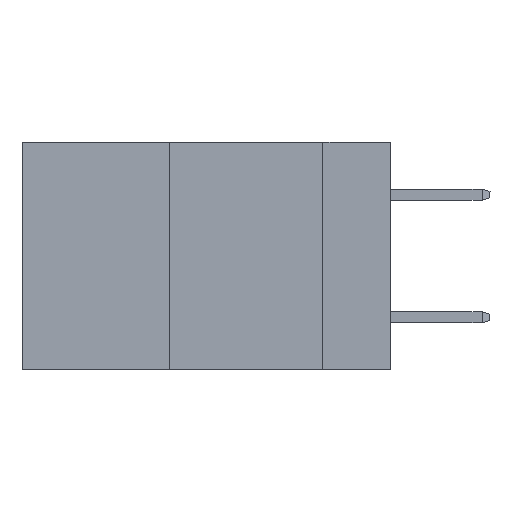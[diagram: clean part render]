
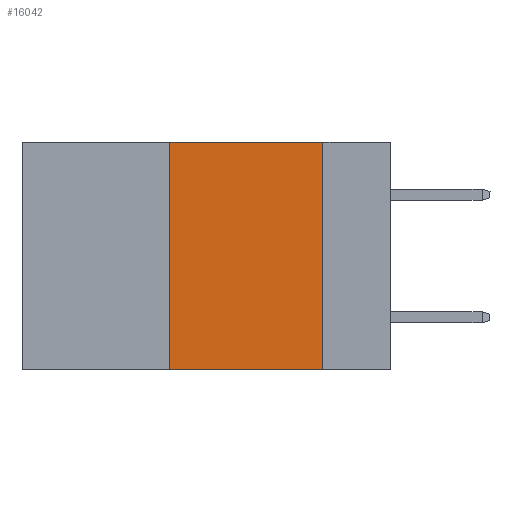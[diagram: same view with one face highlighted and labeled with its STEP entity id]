
A CAD part, left-side view. The second image highlights one B-rep face of the part: STEP entity #16042.
In plain terms, the highlighted planar face has unit normal (-1, 0, 0).
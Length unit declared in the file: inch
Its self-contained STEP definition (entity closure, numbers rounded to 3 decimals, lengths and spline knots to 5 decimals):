
#69 = AXIS2_PLACEMENT_3D ( 'NONE', #8861, #10184, #2370 ) ;
#416 = DIRECTION ( 'NONE',  ( 0., -1., 0. ) ) ;
#794 = CARTESIAN_POINT ( 'NONE',  ( 0., 0.6, -0.37 ) ) ;
#1699 = CARTESIAN_POINT ( 'NONE',  ( 0., 0.36, 0. ) ) ;
#1700 = CARTESIAN_POINT ( 'NONE',  ( 0., 0.36, 0. ) ) ;
#2370 = DIRECTION ( 'NONE',  ( 0., 0., -1. ) ) ;
#2423 = VERTEX_POINT ( 'NONE', #6934 ) ;
#4205 = EDGE_CURVE ( 'NONE', #4821, #9340, #15015, .T. ) ;
#4734 = FACE_OUTER_BOUND ( 'NONE', #6098, .T. ) ;
#4821 = VERTEX_POINT ( 'NONE', #1699 ) ;
#5469 = EDGE_CURVE ( 'NONE', #9340, #2423, #13984, .T. ) ;
#5676 = EDGE_CURVE ( 'NONE', #10452, #2423, #8193, .T. ) ;
#6098 = EDGE_LOOP ( 'NONE', ( #7276, #10750, #9312, #6688 ) ) ;
#6688 = ORIENTED_EDGE ( 'NONE', *, *, #5676, .T. ) ;
#6934 = CARTESIAN_POINT ( 'NONE',  ( 0., 0.11, -0.37 ) ) ;
#7276 = ORIENTED_EDGE ( 'NONE', *, *, #5469, .F. ) ;
#7585 = VECTOR ( 'NONE', #15922, 39.37008 ) ;
#7773 = VECTOR ( 'NONE', #10014, 39.37008 ) ;
#8193 = LINE ( 'NONE', #794, #7773 ) ;
#8861 = CARTESIAN_POINT ( 'NONE',  ( 0., 0.6, 0. ) ) ;
#9312 = ORIENTED_EDGE ( 'NONE', *, *, #10971, .F. ) ;
#9340 = VERTEX_POINT ( 'NONE', #12831 ) ;
#9648 = CARTESIAN_POINT ( 'NONE',  ( 0., 0.6, 0. ) ) ;
#9767 = CARTESIAN_POINT ( 'NONE',  ( 0., 0.36, -0.37 ) ) ;
#9960 = LINE ( 'NONE', #1700, #10378 ) ;
#10014 = DIRECTION ( 'NONE',  ( 0., -1., 0. ) ) ;
#10184 = DIRECTION ( 'NONE',  ( 1., 0., 0. ) ) ;
#10378 = VECTOR ( 'NONE', #15835, 39.37008 ) ;
#10452 = VERTEX_POINT ( 'NONE', #9767 ) ;
#10750 = ORIENTED_EDGE ( 'NONE', *, *, #4205, .F. ) ;
#10971 = EDGE_CURVE ( 'NONE', #10452, #4821, #9960, .T. ) ;
#12091 = VECTOR ( 'NONE', #416, 39.37008 ) ;
#12831 = CARTESIAN_POINT ( 'NONE',  ( 0., 0.11, 0. ) ) ;
#13470 = CARTESIAN_POINT ( 'NONE',  ( 0., 0.11, 0. ) ) ;
#13984 = LINE ( 'NONE', #13470, #7585 ) ;
#15015 = LINE ( 'NONE', #9648, #12091 ) ;
#15835 = DIRECTION ( 'NONE',  ( 0., 0., 1. ) ) ;
#15922 = DIRECTION ( 'NONE',  ( 0., 0., -1. ) ) ;
#16042 = ADVANCED_FACE ( 'NONE', ( #4734 ), #16459, .F. ) ;
#16459 = PLANE ( 'NONE',  #69 ) ;
